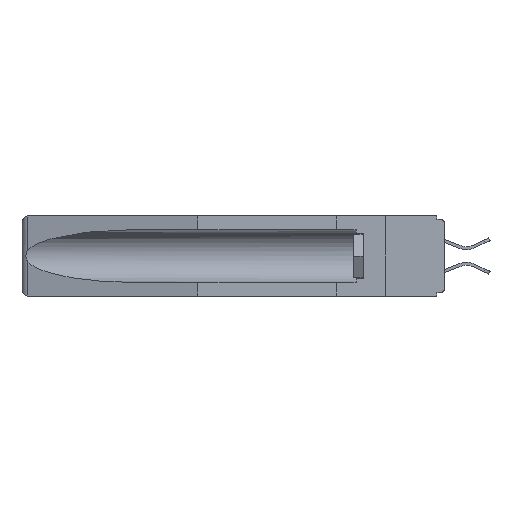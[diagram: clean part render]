
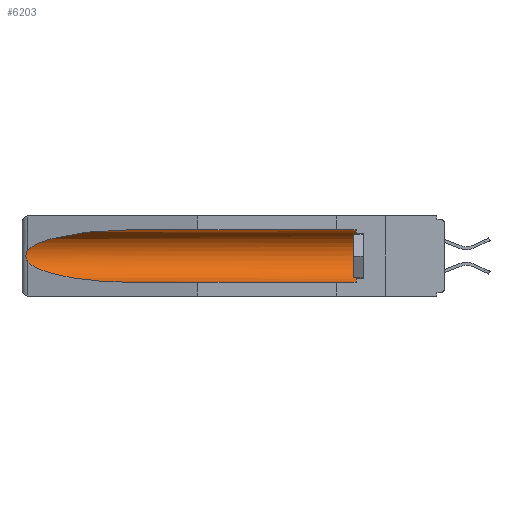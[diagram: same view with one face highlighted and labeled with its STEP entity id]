
A CAD part, left-side view. The second image highlights one B-rep face of the part: STEP entity #6203.
In plain terms, the highlighted cylindrical face has radius 2.857 mm (diameter 5.715 mm), a partial arc.
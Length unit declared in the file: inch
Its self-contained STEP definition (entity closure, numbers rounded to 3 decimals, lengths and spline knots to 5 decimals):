
#646 = FACE_OUTER_BOUND ( 'NONE', #11732, .T. ) ;
#972 = CARTESIAN_POINT ( 'NONE',  ( 0.26597, 1.5296, -0.19026 ) ) ;
#1370 = VERTEX_POINT ( 'NONE', #1576 ) ;
#1399 = CARTESIAN_POINT ( 'NONE',  ( 0.155, -0.30754, -0.1715 ) ) ;
#1576 = CARTESIAN_POINT ( 'NONE',  ( 0.155, 1.07973, -0.284 ) ) ;
#1711 = EDGE_CURVE ( 'NONE', #8824, #9056, #8086, .T. ) ;
#2074 = CARTESIAN_POINT ( 'NONE',  ( 0.26537, 1.52718, -0.14972 ) ) ;
#2161 = CARTESIAN_POINT ( 'NONE',  ( 0.155, -0.30754, -0.284 ) ) ;
#2332 = CARTESIAN_POINT ( 'NONE',  ( 0.25451, 1.48313, -0.09465 ) ) ;
#2338 = CARTESIAN_POINT ( 'NONE',  ( 0.2675, 1.53308, -0.17534 ) ) ;
#2405 = DIRECTION ( 'NONE',  ( 0., 1., 0. ) ) ;
#2462 =( BOUNDED_CURVE ( )  B_SPLINE_CURVE ( 3, ( #9394, #5314, #2332, #13790 ),
 .UNSPECIFIED., .F., .F. ) 
 B_SPLINE_CURVE_WITH_KNOTS ( ( 4, 4 ),
 ( 4.71239, 6.08839 ),
 .UNSPECIFIED. ) 
 CURVE ( )  GEOMETRIC_REPRESENTATION_ITEM ( )  RATIONAL_B_SPLINE_CURVE ( ( 1., 0.848, 0.848, 1. ) ) 
 REPRESENTATION_ITEM ( '' )  );
#2506 = ORIENTED_EDGE ( 'NONE', *, *, #6508, .T. ) ;
#2522 = CARTESIAN_POINT ( 'NONE',  ( 0.155, 1.07973, -0.059 ) ) ;
#2731 = VECTOR ( 'NONE', #16137, 39.37008 ) ;
#2775 = CARTESIAN_POINT ( 'NONE',  ( 0.155, 0.126, -0.1715 ) ) ;
#2800 = CYLINDRICAL_SURFACE ( 'NONE', #9968, 0.1125 ) ;
#2925 = DIRECTION ( 'NONE',  ( 0., 0., 1. ) ) ;
#3138 = ORIENTED_EDGE ( 'NONE', *, *, #11177, .F. ) ;
#3217 = VERTEX_POINT ( 'NONE', #3248 ) ;
#3248 = CARTESIAN_POINT ( 'NONE',  ( 0.155, 0.126, -0.284 ) ) ;
#3317 = EDGE_CURVE ( 'NONE', #8107, #1370, #9126, .T. ) ;
#3779 = VECTOR ( 'NONE', #2405, 39.37008 ) ;
#4152 = CARTESIAN_POINT ( 'NONE',  ( 0.21114, 1.30732, -0.284 ) ) ;
#4411 = DIRECTION ( 'NONE',  ( 0., 1., 0. ) ) ;
#5062 = CARTESIAN_POINT ( 'NONE',  ( 0.26537, 1.52718, -0.19328 ) ) ;
#5314 = CARTESIAN_POINT ( 'NONE',  ( 0.21114, 1.30732, -0.059 ) ) ;
#5550 = LINE ( 'NONE', #2161, #3779 ) ;
#6203 = ADVANCED_FACE ( 'NONE', ( #646 ), #2800, .F. ) ;
#6455 = CIRCLE ( 'NONE', #14016, 0.1125 ) ;
#6503 = CARTESIAN_POINT ( 'NONE',  ( 0.2673, 1.5327, -0.16383 ) ) ;
#6508 = EDGE_CURVE ( 'NONE', #9056, #10398, #2462, .T. ) ;
#6678 = EDGE_CURVE ( 'NONE', #3217, #8824, #6455, .T. ) ;
#7067 = CARTESIAN_POINT ( 'NONE',  ( 0.25451, 1.48313, -0.24835 ) ) ;
#8086 = LINE ( 'NONE', #14806, #2731 ) ;
#8107 = VERTEX_POINT ( 'NONE', #8309 ) ;
#8309 = CARTESIAN_POINT ( 'NONE',  ( 0.26537, 1.52718, -0.19328 ) ) ;
#8824 = VERTEX_POINT ( 'NONE', #11957 ) ;
#9056 = VERTEX_POINT ( 'NONE', #2522 ) ;
#9126 =( BOUNDED_CURVE ( )  B_SPLINE_CURVE ( 3, ( #14124, #7067, #4152, #12767 ),
 .UNSPECIFIED., .F., .F. ) 
 B_SPLINE_CURVE_WITH_KNOTS ( ( 4, 4 ),
 ( 0.1948, 1.5708 ),
 .UNSPECIFIED. ) 
 CURVE ( )  GEOMETRIC_REPRESENTATION_ITEM ( )  RATIONAL_B_SPLINE_CURVE ( ( 1., 0.848, 0.848, 1. ) ) 
 REPRESENTATION_ITEM ( '' )  );
#9394 = CARTESIAN_POINT ( 'NONE',  ( 0.155, 1.07973, -0.059 ) ) ;
#9968 = AXIS2_PLACEMENT_3D ( 'NONE', #1399, #4411, #2925 ) ;
#10398 = VERTEX_POINT ( 'NONE', #2074 ) ;
#11177 = EDGE_CURVE ( 'NONE', #3217, #1370, #5550, .T. ) ;
#11203 = EDGE_CURVE ( 'NONE', #10398, #8107, #11506, .T. ) ;
#11318 = ORIENTED_EDGE ( 'NONE', *, *, #11203, .T. ) ;
#11392 = DIRECTION ( 'NONE',  ( 0., 0., 1. ) ) ;
#11506 = B_SPLINE_CURVE_WITH_KNOTS ( 'NONE', 3,
 ( #13618, #13502, #17960, #6503, #14921, #2338, #13738, #12156, #972, #5062 ),
 .UNSPECIFIED., .F., .F.,
 ( 4, 2, 2, 2, 4 ),
 ( 0., 0.00029, 0.00058, 0.00087, 0.00117 ),
 .UNSPECIFIED. ) ;
#11732 = EDGE_LOOP ( 'NONE', ( #2506, #11318, #16944, #3138, #13819, #13000 ) ) ;
#11957 = CARTESIAN_POINT ( 'NONE',  ( 0.155, 0.126, -0.059 ) ) ;
#12156 = CARTESIAN_POINT ( 'NONE',  ( 0.26655, 1.53094, -0.18657 ) ) ;
#12767 = CARTESIAN_POINT ( 'NONE',  ( 0.155, 1.07973, -0.284 ) ) ;
#13000 = ORIENTED_EDGE ( 'NONE', *, *, #1711, .T. ) ;
#13502 = CARTESIAN_POINT ( 'NONE',  ( 0.26597, 1.52961, -0.15275 ) ) ;
#13618 = CARTESIAN_POINT ( 'NONE',  ( 0.26537, 1.52718, -0.14972 ) ) ;
#13738 = CARTESIAN_POINT ( 'NONE',  ( 0.2673, 1.53269, -0.17917 ) ) ;
#13790 = CARTESIAN_POINT ( 'NONE',  ( 0.26537, 1.52718, -0.14972 ) ) ;
#13819 = ORIENTED_EDGE ( 'NONE', *, *, #6678, .T. ) ;
#14016 = AXIS2_PLACEMENT_3D ( 'NONE', #2775, #18331, #11392 ) ;
#14124 = CARTESIAN_POINT ( 'NONE',  ( 0.26537, 1.52718, -0.19328 ) ) ;
#14806 = CARTESIAN_POINT ( 'NONE',  ( 0.155, -0.30754, -0.059 ) ) ;
#14921 = CARTESIAN_POINT ( 'NONE',  ( 0.2675, 1.53308, -0.16763 ) ) ;
#16137 = DIRECTION ( 'NONE',  ( 0., 1., 0. ) ) ;
#16944 = ORIENTED_EDGE ( 'NONE', *, *, #3317, .T. ) ;
#17960 = CARTESIAN_POINT ( 'NONE',  ( 0.26654, 1.53092, -0.15636 ) ) ;
#18331 = DIRECTION ( 'NONE',  ( 0., -1., 0. ) ) ;
